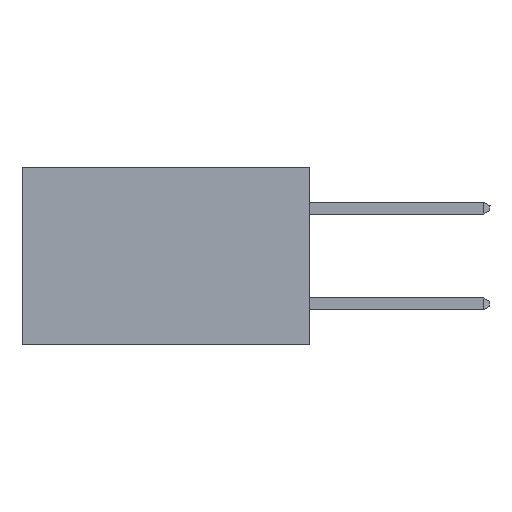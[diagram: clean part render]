
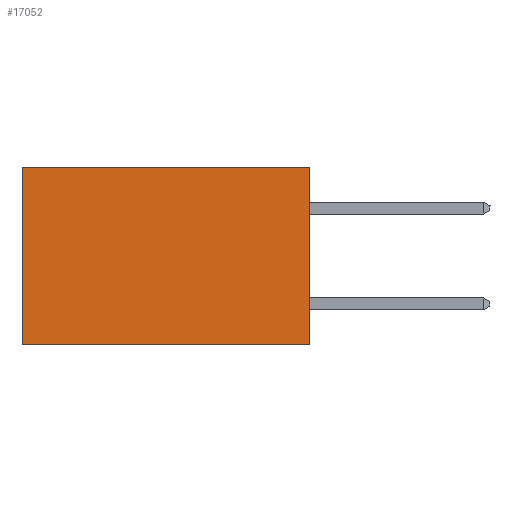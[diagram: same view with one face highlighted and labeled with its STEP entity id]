
A CAD part, left-side view. The second image highlights one B-rep face of the part: STEP entity #17052.
In plain terms, the highlighted planar face has unit normal (-1, 0, 0).
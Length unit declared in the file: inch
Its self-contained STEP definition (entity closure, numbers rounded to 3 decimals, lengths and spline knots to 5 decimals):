
#122 = LINE ( 'NONE', #20042, #2636 ) ;
#1716 = CARTESIAN_POINT ( 'NONE',  ( 0.2875, 0., -0.37 ) ) ;
#1868 = VERTEX_POINT ( 'NONE', #22873 ) ;
#2636 = VECTOR ( 'NONE', #10191, 39.37008 ) ;
#2928 = DIRECTION ( 'NONE',  ( 0., 0., -1. ) ) ;
#3140 = LINE ( 'NONE', #5643, #19328 ) ;
#3421 = CARTESIAN_POINT ( 'NONE',  ( 0.2875, 0., 0. ) ) ;
#3535 = DIRECTION ( 'NONE',  ( 1., 0., 0. ) ) ;
#4264 = EDGE_CURVE ( 'NONE', #12986, #1868, #3140, .T. ) ;
#5643 = CARTESIAN_POINT ( 'NONE',  ( 0.2875, 0., -0.37 ) ) ;
#6297 = CARTESIAN_POINT ( 'NONE',  ( 0.2875, 0., 0. ) ) ;
#8668 = PLANE ( 'NONE',  #19554 ) ;
#8862 = FACE_OUTER_BOUND ( 'NONE', #18941, .T. ) ;
#9386 = LINE ( 'NONE', #6297, #22047 ) ;
#9463 = ORIENTED_EDGE ( 'NONE', *, *, #19654, .T. ) ;
#10191 = DIRECTION ( 'NONE',  ( 0., 0., -1. ) ) ;
#10319 = DIRECTION ( 'NONE',  ( 0., 1., 0. ) ) ;
#11078 = ORIENTED_EDGE ( 'NONE', *, *, #4264, .F. ) ;
#12986 = VERTEX_POINT ( 'NONE', #1716 ) ;
#13859 = EDGE_CURVE ( 'NONE', #22943, #1868, #122, .T. ) ;
#14773 = VERTEX_POINT ( 'NONE', #3421 ) ;
#15680 = DIRECTION ( 'NONE',  ( 0., 1., 0. ) ) ;
#17052 = ADVANCED_FACE ( 'NONE', ( #8862 ), #8668, .F. ) ;
#18135 = ORIENTED_EDGE ( 'NONE', *, *, #18918, .F. ) ;
#18278 = LINE ( 'NONE', #20086, #21055 ) ;
#18918 = EDGE_CURVE ( 'NONE', #14773, #12986, #9386, .T. ) ;
#18941 = EDGE_LOOP ( 'NONE', ( #23879, #11078, #18135, #9463 ) ) ;
#19328 = VECTOR ( 'NONE', #15680, 39.37008 ) ;
#19554 = AXIS2_PLACEMENT_3D ( 'NONE', #20504, #3535, #2928 ) ;
#19654 = EDGE_CURVE ( 'NONE', #14773, #22943, #18278, .T. ) ;
#19788 = CARTESIAN_POINT ( 'NONE',  ( 0.2875, 0.6, 0. ) ) ;
#20042 = CARTESIAN_POINT ( 'NONE',  ( 0.2875, 0.6, 0. ) ) ;
#20086 = CARTESIAN_POINT ( 'NONE',  ( 0.2875, 0., 0. ) ) ;
#20504 = CARTESIAN_POINT ( 'NONE',  ( 0.2875, 0., 0. ) ) ;
#21055 = VECTOR ( 'NONE', #10319, 39.37008 ) ;
#22047 = VECTOR ( 'NONE', #22178, 39.37008 ) ;
#22178 = DIRECTION ( 'NONE',  ( 0., 0., -1. ) ) ;
#22873 = CARTESIAN_POINT ( 'NONE',  ( 0.2875, 0.6, -0.37 ) ) ;
#22943 = VERTEX_POINT ( 'NONE', #19788 ) ;
#23879 = ORIENTED_EDGE ( 'NONE', *, *, #13859, .T. ) ;
